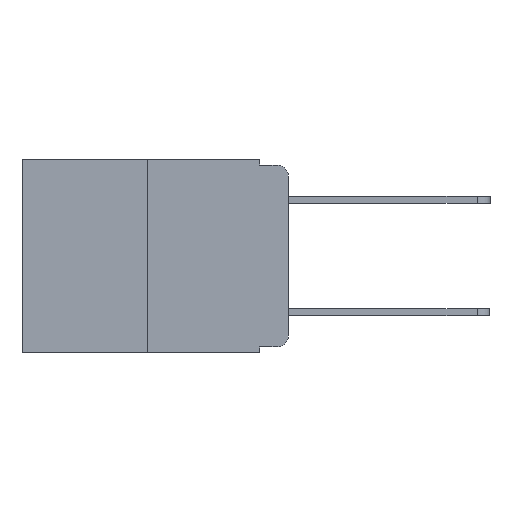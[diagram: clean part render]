
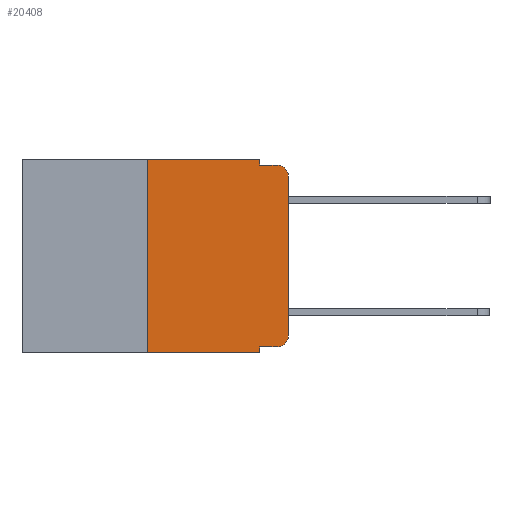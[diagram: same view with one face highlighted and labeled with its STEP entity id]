
A CAD part, left-side view. The second image highlights one B-rep face of the part: STEP entity #20408.
In plain terms, the highlighted planar face has unit normal (-1, 0, 0).
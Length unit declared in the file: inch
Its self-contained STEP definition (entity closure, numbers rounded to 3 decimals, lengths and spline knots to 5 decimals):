
#147 = VERTEX_POINT ( 'NONE', #6941 ) ;
#189 = EDGE_CURVE ( 'NONE', #17988, #19688, #2338, .T. ) ;
#203 = LINE ( 'NONE', #18371, #23242 ) ;
#211 = DIRECTION ( 'NONE',  ( 0., 0., -1. ) ) ;
#742 = LINE ( 'NONE', #12694, #9950 ) ;
#1408 = EDGE_CURVE ( 'NONE', #15089, #11339, #15910, .T. ) ;
#1554 = EDGE_CURVE ( 'NONE', #147, #18655, #2267, .T. ) ;
#1971 = CARTESIAN_POINT ( 'NONE',  ( 0., 0.473, 0. ) ) ;
#2257 = ORIENTED_EDGE ( 'NONE', *, *, #21571, .F. ) ;
#2267 = LINE ( 'NONE', #14322, #21003 ) ;
#2330 = VERTEX_POINT ( 'NONE', #3305 ) ;
#2338 = LINE ( 'NONE', #4930, #16250 ) ;
#2723 = VERTEX_POINT ( 'NONE', #22428 ) ;
#2739 = DIRECTION ( 'NONE',  ( -1., 0., 0. ) ) ;
#3260 = VERTEX_POINT ( 'NONE', #17156 ) ;
#3275 = EDGE_LOOP ( 'NONE', ( #14666, #7217, #2257, #10345, #5049, #15291, #16742, #14268, #20073, #21960 ) ) ;
#3305 = CARTESIAN_POINT ( 'NONE',  ( 0., 0.25, -0.343 ) ) ;
#3699 = CARTESIAN_POINT ( 'NONE',  ( 0., 0., -0.03 ) ) ;
#3827 = PLANE ( 'NONE',  #22346 ) ;
#4394 = CARTESIAN_POINT ( 'NONE',  ( 0., 0.02, -0.03 ) ) ;
#4748 = CARTESIAN_POINT ( 'NONE',  ( 0., 0.02, -0.333 ) ) ;
#4930 = CARTESIAN_POINT ( 'NONE',  ( 0., 0., 0. ) ) ;
#5049 = ORIENTED_EDGE ( 'NONE', *, *, #18876, .F. ) ;
#5057 = CIRCLE ( 'NONE', #15532, 0.02 ) ;
#5280 = VECTOR ( 'NONE', #13549, 39.37008 ) ;
#5382 = CARTESIAN_POINT ( 'NONE',  ( 0., 0.25, 0. ) ) ;
#5623 = CARTESIAN_POINT ( 'NONE',  ( 0., 0., -0.313 ) ) ;
#5674 = DIRECTION ( 'NONE',  ( 1., 0., 0. ) ) ;
#6235 = DIRECTION ( 'NONE',  ( 0., 0., -1. ) ) ;
#6941 = CARTESIAN_POINT ( 'NONE',  ( 0., 0.051, 0. ) ) ;
#7217 = ORIENTED_EDGE ( 'NONE', *, *, #17042, .T. ) ;
#7332 = LINE ( 'NONE', #22008, #7906 ) ;
#7724 = EDGE_CURVE ( 'NONE', #2330, #19608, #8025, .T. ) ;
#7906 = VECTOR ( 'NONE', #211, 39.37008 ) ;
#8025 = LINE ( 'NONE', #16952, #12281 ) ;
#8746 = DIRECTION ( 'NONE',  ( 0., 0., 1. ) ) ;
#9196 = EDGE_CURVE ( 'NONE', #2330, #3260, #742, .T. ) ;
#9950 = VECTOR ( 'NONE', #23527, 39.37008 ) ;
#10345 = ORIENTED_EDGE ( 'NONE', *, *, #1554, .F. ) ;
#10942 = CARTESIAN_POINT ( 'NONE',  ( 0., 0.051, -0.333 ) ) ;
#11339 = VERTEX_POINT ( 'NONE', #4748 ) ;
#11434 = AXIS2_PLACEMENT_3D ( 'NONE', #13658, #2739, #15443 ) ;
#11813 = CARTESIAN_POINT ( 'NONE',  ( 0., 0.051, -0.333 ) ) ;
#12281 = VECTOR ( 'NONE', #22297, 39.37008 ) ;
#12694 = CARTESIAN_POINT ( 'NONE',  ( 0., 0.473, -0.343 ) ) ;
#13549 = DIRECTION ( 'NONE',  ( 0., -1., 0. ) ) ;
#13658 = CARTESIAN_POINT ( 'NONE',  ( 0., 0.02, -0.313 ) ) ;
#14185 = DIRECTION ( 'NONE',  ( 0., -1., 0. ) ) ;
#14268 = ORIENTED_EDGE ( 'NONE', *, *, #17418, .F. ) ;
#14322 = CARTESIAN_POINT ( 'NONE',  ( 0., 0.051, 0. ) ) ;
#14666 = ORIENTED_EDGE ( 'NONE', *, *, #189, .T. ) ;
#14736 = EDGE_CURVE ( 'NONE', #11339, #17988, #20476, .T. ) ;
#15089 = VERTEX_POINT ( 'NONE', #10942 ) ;
#15291 = ORIENTED_EDGE ( 'NONE', *, *, #7724, .F. ) ;
#15391 = DIRECTION ( 'NONE',  ( 0., 0., -1. ) ) ;
#15443 = DIRECTION ( 'NONE',  ( 0., 0., -1. ) ) ;
#15532 = AXIS2_PLACEMENT_3D ( 'NONE', #4394, #17071, #6235 ) ;
#15910 = LINE ( 'NONE', #11813, #19586 ) ;
#16250 = VECTOR ( 'NONE', #8746, 39.37008 ) ;
#16619 = LINE ( 'NONE', #18967, #5280 ) ;
#16742 = ORIENTED_EDGE ( 'NONE', *, *, #9196, .T. ) ;
#16952 = CARTESIAN_POINT ( 'NONE',  ( 0., 0.25, 0. ) ) ;
#17042 = EDGE_CURVE ( 'NONE', #19688, #2723, #5057, .T. ) ;
#17071 = DIRECTION ( 'NONE',  ( -1., 0., 0. ) ) ;
#17156 = CARTESIAN_POINT ( 'NONE',  ( 0., 0.051, -0.343 ) ) ;
#17418 = EDGE_CURVE ( 'NONE', #15089, #3260, #7332, .T. ) ;
#17988 = VERTEX_POINT ( 'NONE', #5623 ) ;
#18338 = DIRECTION ( 'NONE',  ( 0., 0., -1. ) ) ;
#18371 = CARTESIAN_POINT ( 'NONE',  ( 0., 0.051, -0.01 ) ) ;
#18655 = VERTEX_POINT ( 'NONE', #21962 ) ;
#18803 = FACE_OUTER_BOUND ( 'NONE', #3275, .T. ) ;
#18876 = EDGE_CURVE ( 'NONE', #19608, #147, #16619, .T. ) ;
#18967 = CARTESIAN_POINT ( 'NONE',  ( 0., 0.473, 0. ) ) ;
#19586 = VECTOR ( 'NONE', #14185, 39.37008 ) ;
#19608 = VERTEX_POINT ( 'NONE', #5382 ) ;
#19688 = VERTEX_POINT ( 'NONE', #3699 ) ;
#20073 = ORIENTED_EDGE ( 'NONE', *, *, #1408, .T. ) ;
#20170 = DIRECTION ( 'NONE',  ( 0., -1., 0. ) ) ;
#20408 = ADVANCED_FACE ( 'NONE', ( #18803 ), #3827, .F. ) ;
#20476 = CIRCLE ( 'NONE', #11434, 0.02 ) ;
#21003 = VECTOR ( 'NONE', #15391, 39.37008 ) ;
#21571 = EDGE_CURVE ( 'NONE', #18655, #2723, #203, .T. ) ;
#21960 = ORIENTED_EDGE ( 'NONE', *, *, #14736, .T. ) ;
#21962 = CARTESIAN_POINT ( 'NONE',  ( 0., 0.051, -0.01 ) ) ;
#22008 = CARTESIAN_POINT ( 'NONE',  ( 0., 0.051, 0. ) ) ;
#22297 = DIRECTION ( 'NONE',  ( 0., 0., 1. ) ) ;
#22346 = AXIS2_PLACEMENT_3D ( 'NONE', #1971, #5674, #18338 ) ;
#22428 = CARTESIAN_POINT ( 'NONE',  ( 0., 0.02, -0.01 ) ) ;
#23242 = VECTOR ( 'NONE', #20170, 39.37008 ) ;
#23527 = DIRECTION ( 'NONE',  ( 0., -1., 0. ) ) ;
